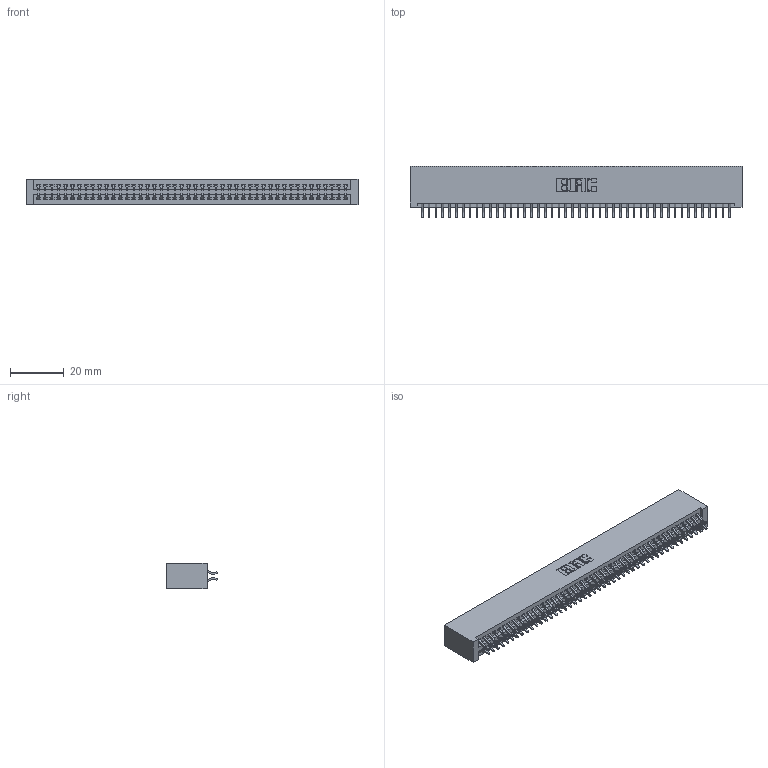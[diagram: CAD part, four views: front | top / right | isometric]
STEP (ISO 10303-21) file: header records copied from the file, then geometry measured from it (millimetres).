
FILE_DESCRIPTION (( 'STEP AP203' ), '1' );
FILE_NAME ('345-092-556-201.STEP', '2019-11-01T20:41:35', ( '' ), ( '' ), 'SwSTEP 2.0', 'SolidWorks 2016', '' );
FILE_SCHEMA (( 'CONFIG_CONTROL_DESIGN' ));
Length unit declared in the file: inch
Products named in the file (3): 345-092-556-201; 345-292-001_556 Tail; 345 Part_No Mounting Lugs
Assembly tree (93 placements, depth 2):
  345-092-556-201
    345 Part_No Mounting Lugs
    345-292-001_556 Tail  x92
Bounding box: 123.44 x 19.24 x 9.4 mm (x, y, z)
Volume: 12640.9 mm3; surface area: 18985.5 mm2
Topology: 93 solids, 93 shells, 5270 faces, 15681 edges, 10330 vertices
Faces by surface type: plane 3480, cylinder 1790
Entity records: 35497 total; most frequent: CARTESIAN_POINT 5960, ORIENTED_EDGE 5882, DIRECTION 5233, EDGE_CURVE 2941, LINE 2625, VECTOR 2625, VERTEX_POINT 1958, AXIS2_PLACEMENT_3D 1304
